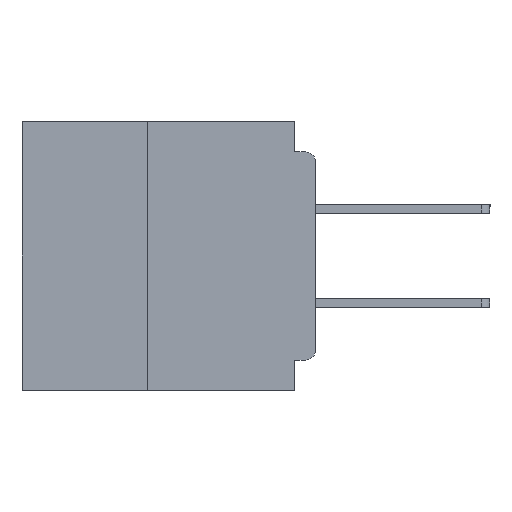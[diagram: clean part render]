
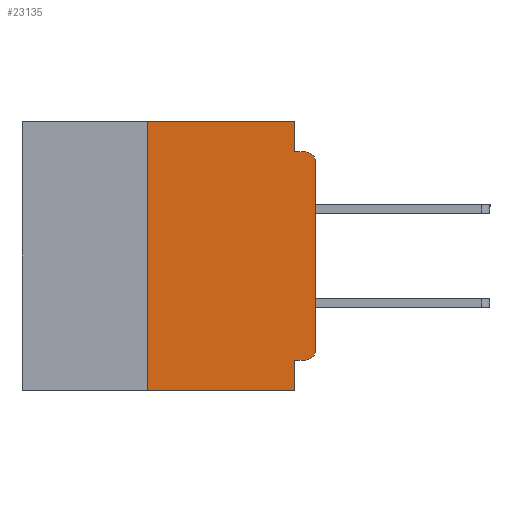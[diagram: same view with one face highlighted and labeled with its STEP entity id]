
A CAD part, left-side view. The second image highlights one B-rep face of the part: STEP entity #23135.
In plain terms, the highlighted planar face has unit normal (-1, 0, 0).
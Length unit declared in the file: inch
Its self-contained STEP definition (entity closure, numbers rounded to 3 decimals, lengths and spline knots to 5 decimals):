
#936 = LINE ( 'NONE', #17541, #17762 ) ;
#1156 = VECTOR ( 'NONE', #18033, 39.37008 ) ;
#1385 = ORIENTED_EDGE ( 'NONE', *, *, #15369, .T. ) ;
#2230 = LINE ( 'NONE', #24604, #1156 ) ;
#2918 = VECTOR ( 'NONE', #30531, 39.37008 ) ;
#3314 = LINE ( 'NONE', #35331, #11230 ) ;
#3629 = ORIENTED_EDGE ( 'NONE', *, *, #19996, .F. ) ;
#3647 = DIRECTION ( 'NONE',  ( 1., 0., 0. ) ) ;
#3957 = EDGE_LOOP ( 'NONE', ( #41448, #31497, #31284, #3629, #5100, #16391, #1385, #31530, #20976, #12549 ) ) ;
#3968 = LINE ( 'NONE', #33877, #2918 ) ;
#4010 = AXIS2_PLACEMENT_3D ( 'NONE', #31580, #11524, #34908 ) ;
#5100 = ORIENTED_EDGE ( 'NONE', *, *, #37926, .F. ) ;
#5344 = VECTOR ( 'NONE', #42866, 39.37008 ) ;
#7654 = CARTESIAN_POINT ( 'NONE',  ( 0., 0.25, -0.4 ) ) ;
#8562 = DIRECTION ( 'NONE',  ( 0., 0., 1. ) ) ;
#9524 = CARTESIAN_POINT ( 'NONE',  ( 0., 0.437, 0. ) ) ;
#9643 = EDGE_CURVE ( 'NONE', #34577, #35850, #31676, .T. ) ;
#10811 = VERTEX_POINT ( 'NONE', #31352 ) ;
#11230 = VECTOR ( 'NONE', #8562, 39.37008 ) ;
#11388 = VERTEX_POINT ( 'NONE', #21050 ) ;
#11524 = DIRECTION ( 'NONE',  ( -1., 0., 0. ) ) ;
#11828 = CARTESIAN_POINT ( 'NONE',  ( 0., 0.031, -0.045 ) ) ;
#12315 = LINE ( 'NONE', #37952, #30088 ) ;
#12370 = CARTESIAN_POINT ( 'NONE',  ( 0., 0.015, -0.045 ) ) ;
#12549 = ORIENTED_EDGE ( 'NONE', *, *, #9643, .T. ) ;
#13567 = LINE ( 'NONE', #29457, #30320 ) ;
#15349 = DIRECTION ( 'NONE',  ( -1., 0., 0. ) ) ;
#15369 = EDGE_CURVE ( 'NONE', #11388, #21747, #12315, .T. ) ;
#15618 = CARTESIAN_POINT ( 'NONE',  ( 0., 0.031, -0.355 ) ) ;
#16391 = ORIENTED_EDGE ( 'NONE', *, *, #19210, .F. ) ;
#17541 = CARTESIAN_POINT ( 'NONE',  ( 0., 0., -0.045 ) ) ;
#17762 = VECTOR ( 'NONE', #40906, 39.37008 ) ;
#17940 = DIRECTION ( 'NONE',  ( 0., -1., 0. ) ) ;
#18033 = DIRECTION ( 'NONE',  ( 0., 0., -1. ) ) ;
#18761 = EDGE_CURVE ( 'NONE', #10811, #27371, #19309, .T. ) ;
#19210 = EDGE_CURVE ( 'NONE', #11388, #36628, #40521, .T. ) ;
#19309 = CIRCLE ( 'NONE', #19464, 0.015 ) ;
#19464 = AXIS2_PLACEMENT_3D ( 'NONE', #35361, #15349, #38716 ) ;
#19471 = CARTESIAN_POINT ( 'NONE',  ( 0., 0.25, 0. ) ) ;
#19996 = EDGE_CURVE ( 'NONE', #36279, #29601, #2230, .T. ) ;
#20976 = ORIENTED_EDGE ( 'NONE', *, *, #31807, .F. ) ;
#21050 = CARTESIAN_POINT ( 'NONE',  ( 0., 0.25, -0.4 ) ) ;
#21564 = CARTESIAN_POINT ( 'NONE',  ( 0., 0., -0.34 ) ) ;
#21747 = VERTEX_POINT ( 'NONE', #32661 ) ;
#22146 = LINE ( 'NONE', #9524, #5344 ) ;
#22961 = CARTESIAN_POINT ( 'NONE',  ( 0., 0.015, -0.355 ) ) ;
#23135 = ADVANCED_FACE ( 'NONE', ( #31919 ), #30349, .F. ) ;
#24604 = CARTESIAN_POINT ( 'NONE',  ( 0., 0.031, 0. ) ) ;
#24876 = VECTOR ( 'NONE', #31125, 39.37008 ) ;
#27067 = CARTESIAN_POINT ( 'NONE',  ( 0., 0.031, 0. ) ) ;
#27105 = DIRECTION ( 'NONE',  ( 0., 0., -1. ) ) ;
#27371 = VERTEX_POINT ( 'NONE', #12370 ) ;
#28540 = EDGE_CURVE ( 'NONE', #35850, #10811, #3314, .T. ) ;
#29457 = CARTESIAN_POINT ( 'NONE',  ( 0., 0.031, -0.4 ) ) ;
#29601 = VERTEX_POINT ( 'NONE', #11828 ) ;
#30088 = VECTOR ( 'NONE', #17940, 39.37008 ) ;
#30218 = AXIS2_PLACEMENT_3D ( 'NONE', #37038, #3647, #27105 ) ;
#30320 = VECTOR ( 'NONE', #32842, 39.37008 ) ;
#30349 = PLANE ( 'NONE',  #30218 ) ;
#30531 = DIRECTION ( 'NONE',  ( 0., 1., 0. ) ) ;
#31125 = DIRECTION ( 'NONE',  ( 0., 0., 1. ) ) ;
#31235 = EDGE_CURVE ( 'NONE', #29601, #27371, #936, .T. ) ;
#31284 = ORIENTED_EDGE ( 'NONE', *, *, #31235, .F. ) ;
#31352 = CARTESIAN_POINT ( 'NONE',  ( 0., 0., -0.06 ) ) ;
#31497 = ORIENTED_EDGE ( 'NONE', *, *, #18761, .T. ) ;
#31530 = ORIENTED_EDGE ( 'NONE', *, *, #39818, .F. ) ;
#31580 = CARTESIAN_POINT ( 'NONE',  ( 0., 0.015, -0.34 ) ) ;
#31676 = CIRCLE ( 'NONE', #4010, 0.015 ) ;
#31807 = EDGE_CURVE ( 'NONE', #34577, #39158, #3968, .T. ) ;
#31919 = FACE_OUTER_BOUND ( 'NONE', #3957, .T. ) ;
#32661 = CARTESIAN_POINT ( 'NONE',  ( 0., 0.031, -0.4 ) ) ;
#32842 = DIRECTION ( 'NONE',  ( 0., 0., -1. ) ) ;
#33877 = CARTESIAN_POINT ( 'NONE',  ( 0., 0., -0.355 ) ) ;
#34577 = VERTEX_POINT ( 'NONE', #22961 ) ;
#34908 = DIRECTION ( 'NONE',  ( 0., 0., -1. ) ) ;
#35331 = CARTESIAN_POINT ( 'NONE',  ( 0., 0., 0. ) ) ;
#35361 = CARTESIAN_POINT ( 'NONE',  ( 0., 0.015, -0.06 ) ) ;
#35850 = VERTEX_POINT ( 'NONE', #21564 ) ;
#36279 = VERTEX_POINT ( 'NONE', #27067 ) ;
#36628 = VERTEX_POINT ( 'NONE', #19471 ) ;
#37038 = CARTESIAN_POINT ( 'NONE',  ( 0., 0.437, 0. ) ) ;
#37926 = EDGE_CURVE ( 'NONE', #36628, #36279, #22146, .T. ) ;
#37952 = CARTESIAN_POINT ( 'NONE',  ( 0., 0.437, -0.4 ) ) ;
#38716 = DIRECTION ( 'NONE',  ( 0., 0., -1. ) ) ;
#39158 = VERTEX_POINT ( 'NONE', #15618 ) ;
#39818 = EDGE_CURVE ( 'NONE', #39158, #21747, #13567, .T. ) ;
#40521 = LINE ( 'NONE', #7654, #24876 ) ;
#40906 = DIRECTION ( 'NONE',  ( 0., -1., 0. ) ) ;
#41448 = ORIENTED_EDGE ( 'NONE', *, *, #28540, .T. ) ;
#42866 = DIRECTION ( 'NONE',  ( 0., -1., 0. ) ) ;
